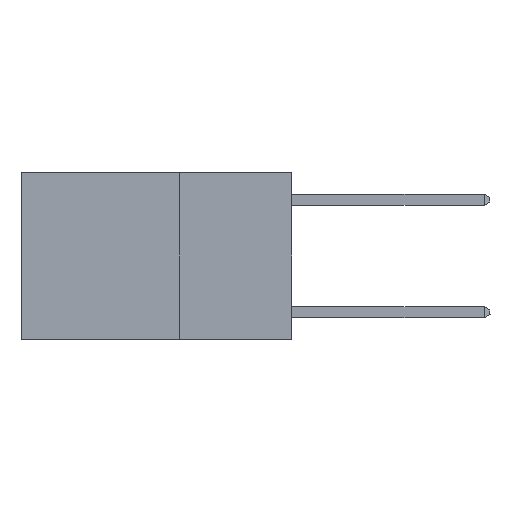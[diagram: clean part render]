
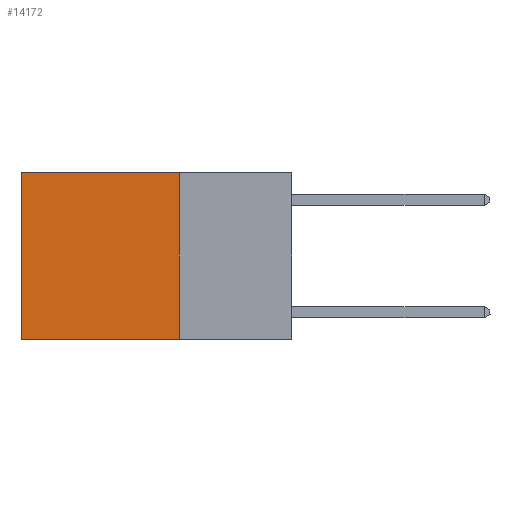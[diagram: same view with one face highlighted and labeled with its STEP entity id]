
A CAD part, left-side view. The second image highlights one B-rep face of the part: STEP entity #14172.
In plain terms, the highlighted planar face has unit normal (-1, 0, 0).
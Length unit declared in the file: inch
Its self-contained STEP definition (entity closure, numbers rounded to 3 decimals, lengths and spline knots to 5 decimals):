
#1241 = EDGE_CURVE ( 'NONE', #11790, #4481, #17164, .T. ) ;
#1672 = CARTESIAN_POINT ( 'NONE',  ( 0.2625, 0.25, 0. ) ) ;
#2005 = AXIS2_PLACEMENT_3D ( 'NONE', #17196, #10309, #17021 ) ;
#2672 = CARTESIAN_POINT ( 'NONE',  ( 0.2625, 0.6, 0. ) ) ;
#3900 = DIRECTION ( 'NONE',  ( 0., 0., -1. ) ) ;
#4161 = LINE ( 'NONE', #9334, #6827 ) ;
#4481 = VERTEX_POINT ( 'NONE', #8902 ) ;
#4612 = VECTOR ( 'NONE', #3900, 39.37008 ) ;
#4998 = PLANE ( 'NONE',  #2005 ) ;
#5007 = CARTESIAN_POINT ( 'NONE',  ( 0.2625, 0.25, -0.37 ) ) ;
#6083 = EDGE_LOOP ( 'NONE', ( #15081, #12756, #14887, #14864 ) ) ;
#6102 = CARTESIAN_POINT ( 'NONE',  ( 0.2625, 0.25, 0. ) ) ;
#6827 = VECTOR ( 'NONE', #16105, 39.37008 ) ;
#8541 = LINE ( 'NONE', #6102, #10139 ) ;
#8902 = CARTESIAN_POINT ( 'NONE',  ( 0.2625, 0.6, -0.37 ) ) ;
#9011 = FACE_OUTER_BOUND ( 'NONE', #6083, .T. ) ;
#9334 = CARTESIAN_POINT ( 'NONE',  ( 0.2625, 0.25, 0. ) ) ;
#10139 = VECTOR ( 'NONE', #15329, 39.37008 ) ;
#10235 = EDGE_CURVE ( 'NONE', #12917, #4481, #11700, .T. ) ;
#10309 = DIRECTION ( 'NONE',  ( 1., 0., 0. ) ) ;
#11700 = LINE ( 'NONE', #5007, #17008 ) ;
#11790 = VERTEX_POINT ( 'NONE', #13503 ) ;
#12756 = ORIENTED_EDGE ( 'NONE', *, *, #10235, .F. ) ;
#12917 = VERTEX_POINT ( 'NONE', #13734 ) ;
#13503 = CARTESIAN_POINT ( 'NONE',  ( 0.2625, 0.6, 0. ) ) ;
#13734 = CARTESIAN_POINT ( 'NONE',  ( 0.2625, 0.25, -0.37 ) ) ;
#13870 = VERTEX_POINT ( 'NONE', #1672 ) ;
#14172 = ADVANCED_FACE ( 'NONE', ( #9011 ), #4998, .F. ) ;
#14864 = ORIENTED_EDGE ( 'NONE', *, *, #16894, .T. ) ;
#14887 = ORIENTED_EDGE ( 'NONE', *, *, #17160, .F. ) ;
#15081 = ORIENTED_EDGE ( 'NONE', *, *, #1241, .T. ) ;
#15329 = DIRECTION ( 'NONE',  ( 0., 1., 0. ) ) ;
#15712 = DIRECTION ( 'NONE',  ( 0., 1., 0. ) ) ;
#16105 = DIRECTION ( 'NONE',  ( 0., 0., -1. ) ) ;
#16894 = EDGE_CURVE ( 'NONE', #13870, #11790, #8541, .T. ) ;
#17008 = VECTOR ( 'NONE', #15712, 39.37008 ) ;
#17021 = DIRECTION ( 'NONE',  ( 0., 0., -1. ) ) ;
#17160 = EDGE_CURVE ( 'NONE', #13870, #12917, #4161, .T. ) ;
#17164 = LINE ( 'NONE', #2672, #4612 ) ;
#17196 = CARTESIAN_POINT ( 'NONE',  ( 0.2625, 0.25, 0. ) ) ;
